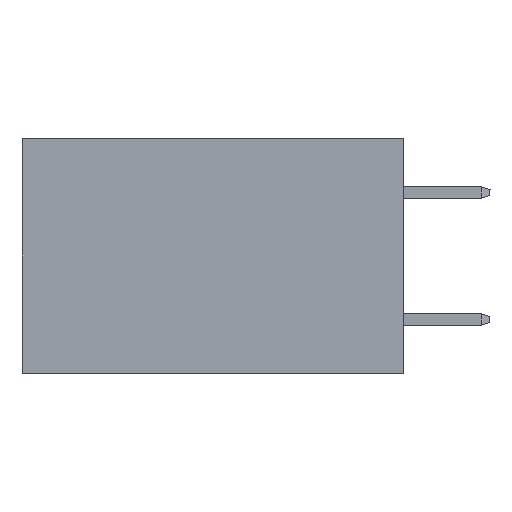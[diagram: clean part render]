
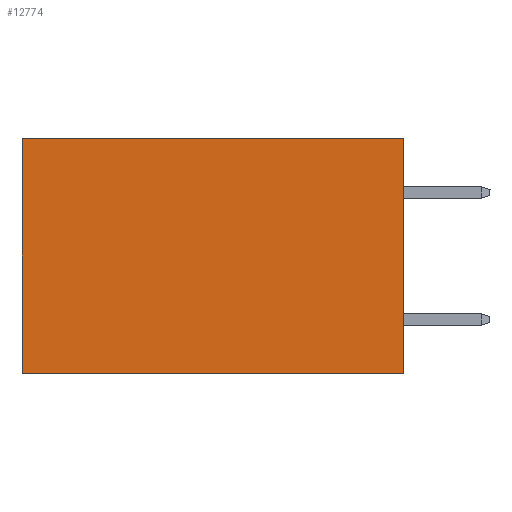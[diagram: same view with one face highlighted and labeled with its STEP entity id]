
A CAD part, left-side view. The second image highlights one B-rep face of the part: STEP entity #12774.
In plain terms, the highlighted planar face has unit normal (-1, 0, 0).
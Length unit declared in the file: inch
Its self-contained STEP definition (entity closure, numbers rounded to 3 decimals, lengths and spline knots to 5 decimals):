
#159 = CARTESIAN_POINT ( 'NONE',  ( 0.2875, 0.6, -0.37 ) ) ;
#1509 = CARTESIAN_POINT ( 'NONE',  ( 0.2875, 0., 0. ) ) ;
#2562 = LINE ( 'NONE', #27256, #17125 ) ;
#2841 = DIRECTION ( 'NONE',  ( 1., 0., 0. ) ) ;
#3374 = CARTESIAN_POINT ( 'NONE',  ( 0.2875, 0., 0. ) ) ;
#4560 = LINE ( 'NONE', #28540, #33223 ) ;
#5398 = CARTESIAN_POINT ( 'NONE',  ( 0.2875, 0., -0.37 ) ) ;
#7243 = LINE ( 'NONE', #1509, #33184 ) ;
#7850 = PLANE ( 'NONE',  #19241 ) ;
#8213 = DIRECTION ( 'NONE',  ( 0., 0., -1. ) ) ;
#8693 = EDGE_CURVE ( 'NONE', #20996, #10865, #2562, .T. ) ;
#10865 = VERTEX_POINT ( 'NONE', #159 ) ;
#11103 = CARTESIAN_POINT ( 'NONE',  ( 0.2875, 0., 0. ) ) ;
#11286 = DIRECTION ( 'NONE',  ( 0., 0., -1. ) ) ;
#12774 = ADVANCED_FACE ( 'NONE', ( #21453 ), #7850, .F. ) ;
#13654 = ORIENTED_EDGE ( 'NONE', *, *, #8693, .F. ) ;
#14002 = CARTESIAN_POINT ( 'NONE',  ( 0.2875, 0.6, 0. ) ) ;
#17125 = VECTOR ( 'NONE', #32667, 39.37008 ) ;
#17797 = DIRECTION ( 'NONE',  ( 0., 0., -1. ) ) ;
#17984 = EDGE_CURVE ( 'NONE', #33779, #10865, #4560, .T. ) ;
#18036 = VERTEX_POINT ( 'NONE', #34112 ) ;
#19241 = AXIS2_PLACEMENT_3D ( 'NONE', #11103, #2841, #8213 ) ;
#20996 = VERTEX_POINT ( 'NONE', #5398 ) ;
#21032 = EDGE_LOOP ( 'NONE', ( #22291, #13654, #24619, #30471 ) ) ;
#21453 = FACE_OUTER_BOUND ( 'NONE', #21032, .T. ) ;
#22291 = ORIENTED_EDGE ( 'NONE', *, *, #17984, .T. ) ;
#24619 = ORIENTED_EDGE ( 'NONE', *, *, #34198, .F. ) ;
#27256 = CARTESIAN_POINT ( 'NONE',  ( 0.2875, 0., -0.37 ) ) ;
#28540 = CARTESIAN_POINT ( 'NONE',  ( 0.2875, 0.6, 0. ) ) ;
#30394 = VECTOR ( 'NONE', #11286, 39.37008 ) ;
#30471 = ORIENTED_EDGE ( 'NONE', *, *, #33019, .T. ) ;
#31955 = DIRECTION ( 'NONE',  ( 0., 1., 0. ) ) ;
#32667 = DIRECTION ( 'NONE',  ( 0., 1., 0. ) ) ;
#32775 = LINE ( 'NONE', #3374, #30394 ) ;
#33019 = EDGE_CURVE ( 'NONE', #18036, #33779, #7243, .T. ) ;
#33184 = VECTOR ( 'NONE', #31955, 39.37008 ) ;
#33223 = VECTOR ( 'NONE', #17797, 39.37008 ) ;
#33779 = VERTEX_POINT ( 'NONE', #14002 ) ;
#34112 = CARTESIAN_POINT ( 'NONE',  ( 0.2875, 0., 0. ) ) ;
#34198 = EDGE_CURVE ( 'NONE', #18036, #20996, #32775, .T. ) ;
